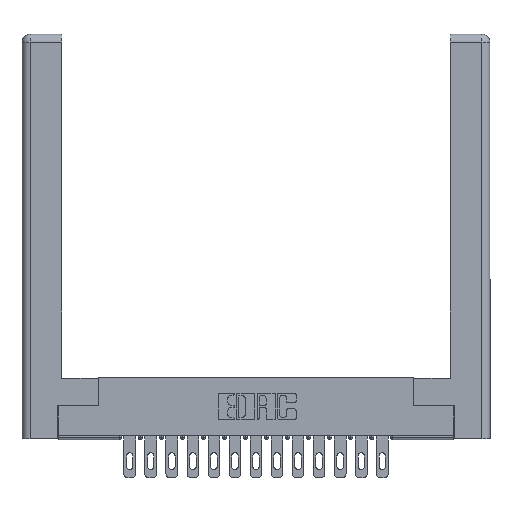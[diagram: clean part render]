
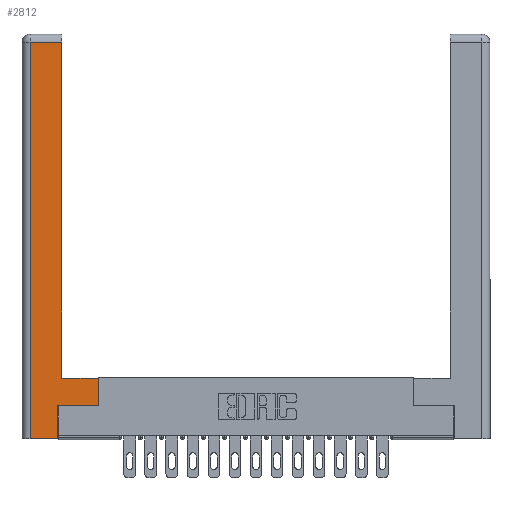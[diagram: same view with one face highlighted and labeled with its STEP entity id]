
A CAD part, top view. The second image highlights one B-rep face of the part: STEP entity #2812.
In plain terms, the highlighted planar face has unit normal (0, 0, 1).
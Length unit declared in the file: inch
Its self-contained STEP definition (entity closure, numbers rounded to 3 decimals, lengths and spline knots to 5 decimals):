
#68 = VERTEX_POINT ( 'NONE', #9050 ) ;
#192 = DIRECTION ( 'NONE',  ( -1., 0., 0. ) ) ;
#343 = VERTEX_POINT ( 'NONE', #6396 ) ;
#425 = VECTOR ( 'NONE', #2207, 39.37008 ) ;
#542 = LINE ( 'NONE', #13323, #14510 ) ;
#649 = VECTOR ( 'NONE', #8031, 39.37008 ) ;
#828 = AXIS2_PLACEMENT_3D ( 'NONE', #11269, #2669, #12718 ) ;
#900 = CARTESIAN_POINT ( 'NONE',  ( 0.295, 0.45, 0. ) ) ;
#909 = EDGE_CURVE ( 'NONE', #343, #18490, #542, .T. ) ;
#933 = VERTEX_POINT ( 'NONE', #13860 ) ;
#1456 = EDGE_CURVE ( 'NONE', #13232, #11721, #5478, .T. ) ;
#2113 = CARTESIAN_POINT ( 'NONE',  ( 0.295, 3., 0. ) ) ;
#2207 = DIRECTION ( 'NONE',  ( 0., 1., 0. ) ) ;
#2500 = LINE ( 'NONE', #17296, #10126 ) ;
#2570 = DIRECTION ( 'NONE',  ( 0., 1., 0. ) ) ;
#2669 = DIRECTION ( 'NONE',  ( 0., 0., -1. ) ) ;
#2812 = ADVANCED_FACE ( 'NONE', ( #7503 ), #11204, .F. ) ;
#2901 = DIRECTION ( 'NONE',  ( 0., -1., 0. ) ) ;
#3109 = CARTESIAN_POINT ( 'NONE',  ( 0.0615, 2.94, 0. ) ) ;
#3308 = ORIENTED_EDGE ( 'NONE', *, *, #1456, .T. ) ;
#3797 = DIRECTION ( 'NONE',  ( 1., 0., 0. ) ) ;
#4243 = EDGE_CURVE ( 'NONE', #11721, #933, #16674, .T. ) ;
#4731 = EDGE_CURVE ( 'NONE', #933, #343, #2500, .T. ) ;
#4816 = ORIENTED_EDGE ( 'NONE', *, *, #7908, .T. ) ;
#5056 = EDGE_CURVE ( 'NONE', #18490, #13519, #8965, .T. ) ;
#5111 = DIRECTION ( 'NONE',  ( 0., 1., 0. ) ) ;
#5203 = VECTOR ( 'NONE', #192, 39.37008 ) ;
#5478 = LINE ( 'NONE', #2113, #8826 ) ;
#6396 = CARTESIAN_POINT ( 'NONE',  ( 0.0615, 0., 0. ) ) ;
#6521 = ORIENTED_EDGE ( 'NONE', *, *, #9341, .T. ) ;
#6839 = EDGE_CURVE ( 'NONE', #10943, #68, #10578, .T. ) ;
#6927 = EDGE_LOOP ( 'NONE', ( #3308, #11549, #8578, #10639, #16343, #6521, #15220, #4816 ) ) ;
#7503 = FACE_OUTER_BOUND ( 'NONE', #6927, .T. ) ;
#7908 = EDGE_CURVE ( 'NONE', #68, #13232, #10753, .T. ) ;
#8031 = DIRECTION ( 'NONE',  ( -1., 0., 0. ) ) ;
#8250 = VECTOR ( 'NONE', #17701, 39.37008 ) ;
#8578 = ORIENTED_EDGE ( 'NONE', *, *, #4731, .T. ) ;
#8826 = VECTOR ( 'NONE', #5111, 39.37008 ) ;
#8965 = LINE ( 'NONE', #10787, #425 ) ;
#9049 = CARTESIAN_POINT ( 'NONE',  ( 0.565, 0.245, 0. ) ) ;
#9050 = CARTESIAN_POINT ( 'NONE',  ( 0.565, 0.45, 0. ) ) ;
#9341 = EDGE_CURVE ( 'NONE', #13519, #10943, #11653, .T. ) ;
#10126 = VECTOR ( 'NONE', #2901, 39.37008 ) ;
#10141 = VECTOR ( 'NONE', #2570, 39.37008 ) ;
#10578 = LINE ( 'NONE', #15427, #10141 ) ;
#10639 = ORIENTED_EDGE ( 'NONE', *, *, #909, .T. ) ;
#10753 = LINE ( 'NONE', #13778, #649 ) ;
#10787 = CARTESIAN_POINT ( 'NONE',  ( 0.265, 0.245, 0. ) ) ;
#10943 = VERTEX_POINT ( 'NONE', #11609 ) ;
#11204 = PLANE ( 'NONE',  #828 ) ;
#11269 = CARTESIAN_POINT ( 'NONE',  ( 0., 0., 0. ) ) ;
#11549 = ORIENTED_EDGE ( 'NONE', *, *, #4243, .T. ) ;
#11609 = CARTESIAN_POINT ( 'NONE',  ( 0.565, 0.245, 0. ) ) ;
#11653 = LINE ( 'NONE', #9049, #8250 ) ;
#11721 = VERTEX_POINT ( 'NONE', #13292 ) ;
#12718 = DIRECTION ( 'NONE',  ( -1., 0., 0. ) ) ;
#13232 = VERTEX_POINT ( 'NONE', #900 ) ;
#13292 = CARTESIAN_POINT ( 'NONE',  ( 0.295, 2.94, 0. ) ) ;
#13323 = CARTESIAN_POINT ( 'NONE',  ( 0.265, 0., 0. ) ) ;
#13357 = CARTESIAN_POINT ( 'NONE',  ( 0.265, 0.245, 0. ) ) ;
#13519 = VERTEX_POINT ( 'NONE', #13357 ) ;
#13778 = CARTESIAN_POINT ( 'NONE',  ( 0.295, 0.45, 0. ) ) ;
#13860 = CARTESIAN_POINT ( 'NONE',  ( 0.0615, 2.94, 0. ) ) ;
#14510 = VECTOR ( 'NONE', #3797, 39.37008 ) ;
#15002 = CARTESIAN_POINT ( 'NONE',  ( 0.265, 0., 0. ) ) ;
#15220 = ORIENTED_EDGE ( 'NONE', *, *, #6839, .T. ) ;
#15427 = CARTESIAN_POINT ( 'NONE',  ( 0.565, 0.45, 0. ) ) ;
#16343 = ORIENTED_EDGE ( 'NONE', *, *, #5056, .T. ) ;
#16674 = LINE ( 'NONE', #3109, #5203 ) ;
#17296 = CARTESIAN_POINT ( 'NONE',  ( 0.0615, 0., 0. ) ) ;
#17701 = DIRECTION ( 'NONE',  ( 1., 0., 0. ) ) ;
#18490 = VERTEX_POINT ( 'NONE', #15002 ) ;
